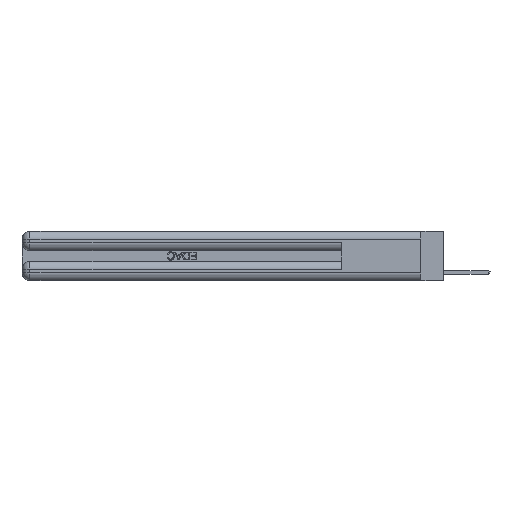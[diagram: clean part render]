
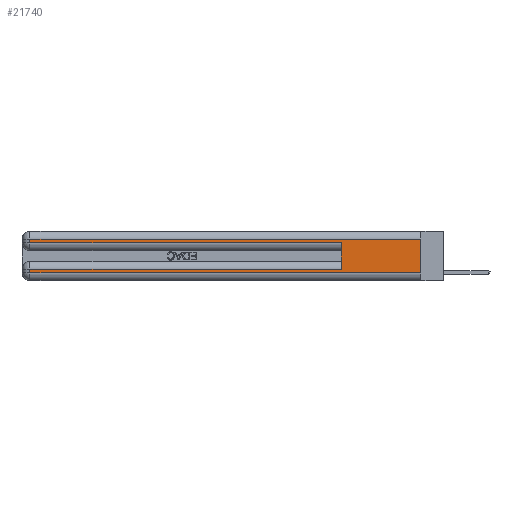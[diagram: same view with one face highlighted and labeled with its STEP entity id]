
A CAD part, left-side view. The second image highlights one B-rep face of the part: STEP entity #21740.
In plain terms, the highlighted planar face has unit normal (-1, 0, 0).
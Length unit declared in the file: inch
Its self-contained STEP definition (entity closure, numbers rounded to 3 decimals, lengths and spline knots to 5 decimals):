
#204 = DIRECTION ( 'NONE',  ( 0., 1., 0. ) ) ;
#514 = ORIENTED_EDGE ( 'NONE', *, *, #11614, .T. ) ;
#928 = ORIENTED_EDGE ( 'NONE', *, *, #24534, .T. ) ;
#994 = VERTEX_POINT ( 'NONE', #26252 ) ;
#1395 = EDGE_CURVE ( 'NONE', #8892, #25420, #22142, .T. ) ;
#1477 = CARTESIAN_POINT ( 'NONE',  ( 0., 0., 0.085 ) ) ;
#1821 = VECTOR ( 'NONE', #10353, 39.37008 ) ;
#1834 = CARTESIAN_POINT ( 'NONE',  ( 0., 0., 0.37 ) ) ;
#2687 = ORIENTED_EDGE ( 'NONE', *, *, #18432, .T. ) ;
#2910 = CARTESIAN_POINT ( 'NONE',  ( 0., 0., 0.31 ) ) ;
#3024 = VECTOR ( 'NONE', #25992, 39.37008 ) ;
#4259 = CARTESIAN_POINT ( 'NONE',  ( 0., 2.94, 0.31 ) ) ;
#5552 = CARTESIAN_POINT ( 'NONE',  ( 0., 2.94, 0.06 ) ) ;
#5860 = LINE ( 'NONE', #15002, #28658 ) ;
#5878 = CARTESIAN_POINT ( 'NONE',  ( 0., 0.6, 0.285 ) ) ;
#5932 = PLANE ( 'NONE',  #16068 ) ;
#6656 = VECTOR ( 'NONE', #19925, 39.37008 ) ;
#6834 = EDGE_CURVE ( 'NONE', #994, #12510, #17204, .T. ) ;
#8675 = DIRECTION ( 'NONE',  ( 0., 0., -1. ) ) ;
#8691 = LINE ( 'NONE', #28351, #3024 ) ;
#8892 = VERTEX_POINT ( 'NONE', #2910 ) ;
#9772 = VECTOR ( 'NONE', #24092, 39.37008 ) ;
#9918 = VECTOR ( 'NONE', #8675, 39.37008 ) ;
#10353 = DIRECTION ( 'NONE',  ( 0., 1., 0. ) ) ;
#10636 = LINE ( 'NONE', #1477, #1821 ) ;
#10990 = CARTESIAN_POINT ( 'NONE',  ( 0., 0., 0.37 ) ) ;
#11614 = EDGE_CURVE ( 'NONE', #994, #23345, #10636, .T. ) ;
#12351 = EDGE_LOOP ( 'NONE', ( #21752, #15957, #928, #23268, #23295, #514, #2687, #16944 ) ) ;
#12510 = VERTEX_POINT ( 'NONE', #5878 ) ;
#12981 = CARTESIAN_POINT ( 'NONE',  ( 0., 0., 0.06 ) ) ;
#13785 = VECTOR ( 'NONE', #20980, 39.37008 ) ;
#14275 = CARTESIAN_POINT ( 'NONE',  ( 0., 0.6, 0.145 ) ) ;
#14677 = VECTOR ( 'NONE', #204, 39.37008 ) ;
#14884 = EDGE_CURVE ( 'NONE', #26487, #25420, #8691, .T. ) ;
#14955 = CARTESIAN_POINT ( 'NONE',  ( 0., 2.94, 0.37 ) ) ;
#15002 = CARTESIAN_POINT ( 'NONE',  ( 0., 0., 0.285 ) ) ;
#15955 = CARTESIAN_POINT ( 'NONE',  ( 0., 0., 0.31 ) ) ;
#15957 = ORIENTED_EDGE ( 'NONE', *, *, #21877, .T. ) ;
#16068 = AXIS2_PLACEMENT_3D ( 'NONE', #10990, #17571, #19908 ) ;
#16944 = ORIENTED_EDGE ( 'NONE', *, *, #14884, .T. ) ;
#17204 = LINE ( 'NONE', #14275, #13785 ) ;
#17571 = DIRECTION ( 'NONE',  ( 1., 0., 0. ) ) ;
#18432 = EDGE_CURVE ( 'NONE', #23345, #26487, #28750, .T. ) ;
#19176 = FACE_OUTER_BOUND ( 'NONE', #12351, .T. ) ;
#19908 = DIRECTION ( 'NONE',  ( 0., 0., -1. ) ) ;
#19925 = DIRECTION ( 'NONE',  ( 0., 0., -1. ) ) ;
#20174 = LINE ( 'NONE', #15955, #14677 ) ;
#20980 = DIRECTION ( 'NONE',  ( 0., 0., 1. ) ) ;
#21527 = LINE ( 'NONE', #14955, #9772 ) ;
#21740 = ADVANCED_FACE ( 'NONE', ( #19176 ), #5932, .F. ) ;
#21752 = ORIENTED_EDGE ( 'NONE', *, *, #1395, .F. ) ;
#21877 = EDGE_CURVE ( 'NONE', #8892, #28779, #20174, .T. ) ;
#22142 = LINE ( 'NONE', #1834, #6656 ) ;
#23268 = ORIENTED_EDGE ( 'NONE', *, *, #27965, .T. ) ;
#23295 = ORIENTED_EDGE ( 'NONE', *, *, #6834, .F. ) ;
#23345 = VERTEX_POINT ( 'NONE', #28499 ) ;
#23991 = DIRECTION ( 'NONE',  ( 0., -1., 0. ) ) ;
#24069 = CARTESIAN_POINT ( 'NONE',  ( 0., 2.94, 0.37 ) ) ;
#24092 = DIRECTION ( 'NONE',  ( 0., 0., -1. ) ) ;
#24534 = EDGE_CURVE ( 'NONE', #28779, #27324, #21527, .T. ) ;
#25420 = VERTEX_POINT ( 'NONE', #12981 ) ;
#25992 = DIRECTION ( 'NONE',  ( 0., -1., 0. ) ) ;
#26151 = CARTESIAN_POINT ( 'NONE',  ( 0., 2.94, 0.285 ) ) ;
#26252 = CARTESIAN_POINT ( 'NONE',  ( 0., 0.6, 0.085 ) ) ;
#26487 = VERTEX_POINT ( 'NONE', #5552 ) ;
#27324 = VERTEX_POINT ( 'NONE', #26151 ) ;
#27965 = EDGE_CURVE ( 'NONE', #27324, #12510, #5860, .T. ) ;
#28351 = CARTESIAN_POINT ( 'NONE',  ( 0., 0., 0.06 ) ) ;
#28499 = CARTESIAN_POINT ( 'NONE',  ( 0., 2.94, 0.085 ) ) ;
#28658 = VECTOR ( 'NONE', #23991, 39.37008 ) ;
#28750 = LINE ( 'NONE', #24069, #9918 ) ;
#28779 = VERTEX_POINT ( 'NONE', #4259 ) ;
